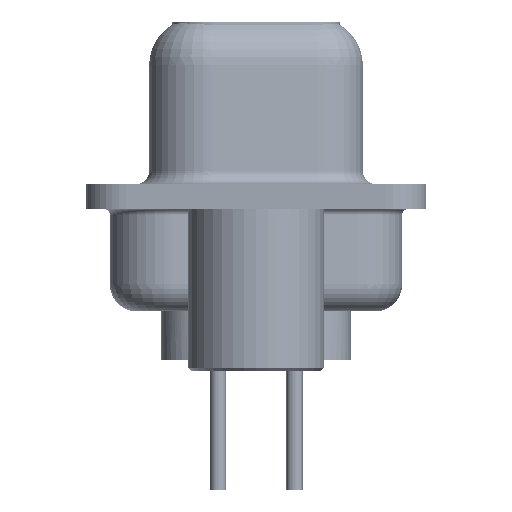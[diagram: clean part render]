
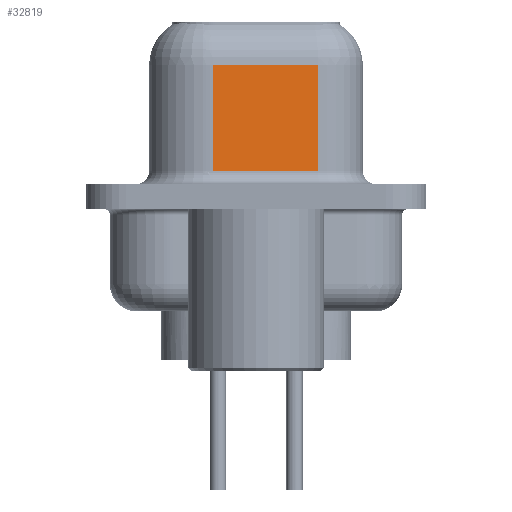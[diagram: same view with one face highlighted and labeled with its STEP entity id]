
A CAD part, left-side view. The second image highlights one B-rep face of the part: STEP entity #32819.
In plain terms, the highlighted planar face has unit normal (-0.985, -0.174, 0).
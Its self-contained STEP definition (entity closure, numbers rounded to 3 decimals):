
#1909 = DIRECTION ( 'NONE',  ( 0., 0., -1. ) ) ;
#3750 = CARTESIAN_POINT ( 'NONE',  ( 4.38, 1.603, 6.6 ) ) ;
#3772 = LINE ( 'NONE', #32471, #3845 ) ;
#3845 = VECTOR ( 'NONE', #1909, 1000. ) ;
#5154 = VECTOR ( 'NONE', #22145, 1000. ) ;
#5282 = EDGE_LOOP ( 'NONE', ( #33298, #15464, #6091, #13830 ) ) ;
#5712 = PLANE ( 'NONE',  #12005 ) ;
#6091 = ORIENTED_EDGE ( 'NONE', *, *, #31117, .T. ) ;
#10104 = EDGE_CURVE ( 'NONE', #23772, #15105, #14183, .T. ) ;
#10903 = VECTOR ( 'NONE', #20310, 1000. ) ;
#12005 = AXIS2_PLACEMENT_3D ( 'NONE', #31057, #31383, #26015 ) ;
#13152 = FACE_OUTER_BOUND ( 'NONE', #5282, .T. ) ;
#13830 = ORIENTED_EDGE ( 'NONE', *, *, #10104, .T. ) ;
#14068 = DIRECTION ( 'NONE',  ( 0., 0., -1. ) ) ;
#14183 = LINE ( 'NONE', #21817, #5154 ) ;
#15105 = VERTEX_POINT ( 'NONE', #29944 ) ;
#15464 = ORIENTED_EDGE ( 'NONE', *, *, #31322, .T. ) ;
#17924 = CARTESIAN_POINT ( 'NONE',  ( 5.068, -2.297, 4.85 ) ) ;
#18128 = EDGE_CURVE ( 'NONE', #19792, #15105, #3772, .T. ) ;
#19792 = VERTEX_POINT ( 'NONE', #23035 ) ;
#20274 = VERTEX_POINT ( 'NONE', #31414 ) ;
#20310 = DIRECTION ( 'NONE',  ( -0.174, 0.985, 0. ) ) ;
#21817 = CARTESIAN_POINT ( 'NONE',  ( 5.068, -2.297, 0.95 ) ) ;
#22145 = DIRECTION ( 'NONE',  ( 0.174, -0.985, 0. ) ) ;
#23035 = CARTESIAN_POINT ( 'NONE',  ( 5.068, -2.297, 4.85 ) ) ;
#23772 = VERTEX_POINT ( 'NONE', #25072 ) ;
#25072 = CARTESIAN_POINT ( 'NONE',  ( 4.38, 1.603, 0.95 ) ) ;
#26015 = DIRECTION ( 'NONE',  ( -0.174, 0.985, 0. ) ) ;
#27730 = LINE ( 'NONE', #17924, #10903 ) ;
#29944 = CARTESIAN_POINT ( 'NONE',  ( 5.068, -2.297, 0.95 ) ) ;
#30309 = VECTOR ( 'NONE', #14068, 1000. ) ;
#31057 = CARTESIAN_POINT ( 'NONE',  ( 5.068, -2.297, 6.6 ) ) ;
#31117 = EDGE_CURVE ( 'NONE', #20274, #23772, #31959, .T. ) ;
#31322 = EDGE_CURVE ( 'NONE', #19792, #20274, #27730, .T. ) ;
#31383 = DIRECTION ( 'NONE',  ( 0.985, 0.174, 0. ) ) ;
#31414 = CARTESIAN_POINT ( 'NONE',  ( 4.38, 1.603, 4.85 ) ) ;
#31959 = LINE ( 'NONE', #3750, #30309 ) ;
#32471 = CARTESIAN_POINT ( 'NONE',  ( 5.068, -2.297, 6.6 ) ) ;
#32819 = ADVANCED_FACE ( 'NONE', ( #13152 ), #5712, .F. ) ;
#33298 = ORIENTED_EDGE ( 'NONE', *, *, #18128, .F. ) ;
